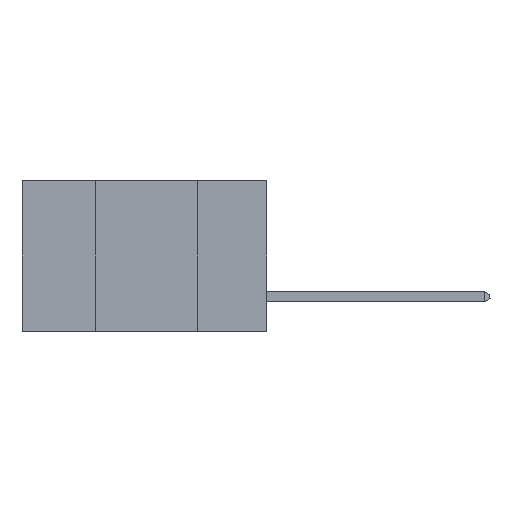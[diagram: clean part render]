
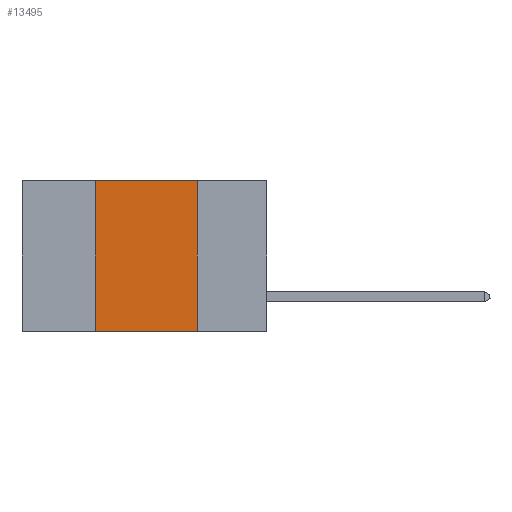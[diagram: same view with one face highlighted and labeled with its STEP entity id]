
A CAD part, left-side view. The second image highlights one B-rep face of the part: STEP entity #13495.
In plain terms, the highlighted planar face has unit normal (-1, 0, 0).
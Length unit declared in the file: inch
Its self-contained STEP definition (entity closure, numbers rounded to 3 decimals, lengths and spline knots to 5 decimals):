
#2422 = LINE ( 'NONE', #14646, #25471 ) ;
#2868 = CARTESIAN_POINT ( 'NONE',  ( 0., 0.42, 0. ) ) ;
#5227 = DIRECTION ( 'NONE',  ( 0., 0., -1. ) ) ;
#6954 = ORIENTED_EDGE ( 'NONE', *, *, #23895, .F. ) ;
#7802 = VERTEX_POINT ( 'NONE', #35195 ) ;
#7934 = EDGE_CURVE ( 'NONE', #14962, #7802, #11717, .T. ) ;
#8700 = DIRECTION ( 'NONE',  ( 0., 0., -1. ) ) ;
#10096 = CARTESIAN_POINT ( 'NONE',  ( 0., 0.42, -0.37 ) ) ;
#11717 = LINE ( 'NONE', #23945, #12528 ) ;
#12528 = VECTOR ( 'NONE', #8700, 39.37008 ) ;
#13495 = ADVANCED_FACE ( 'NONE', ( #26671 ), #35683, .F. ) ;
#14646 = CARTESIAN_POINT ( 'NONE',  ( 0., 0.6, 0. ) ) ;
#14962 = VERTEX_POINT ( 'NONE', #21845 ) ;
#15975 = LINE ( 'NONE', #31417, #37456 ) ;
#17868 = CARTESIAN_POINT ( 'NONE',  ( 0., 0.42, 0. ) ) ;
#18781 = DIRECTION ( 'NONE',  ( 0., -1., 0. ) ) ;
#21075 = DIRECTION ( 'NONE',  ( 0., 0., 1. ) ) ;
#21845 = CARTESIAN_POINT ( 'NONE',  ( 0., 0.17, 0. ) ) ;
#22708 = EDGE_CURVE ( 'NONE', #36100, #7802, #15975, .T. ) ;
#23895 = EDGE_CURVE ( 'NONE', #38594, #14962, #2422, .T. ) ;
#23945 = CARTESIAN_POINT ( 'NONE',  ( 0., 0.17, 0. ) ) ;
#24073 = LINE ( 'NONE', #17868, #25766 ) ;
#25471 = VECTOR ( 'NONE', #26886, 39.37008 ) ;
#25766 = VECTOR ( 'NONE', #21075, 39.37008 ) ;
#26671 = FACE_OUTER_BOUND ( 'NONE', #33852, .T. ) ;
#26886 = DIRECTION ( 'NONE',  ( 0., -1., 0. ) ) ;
#26967 = ORIENTED_EDGE ( 'NONE', *, *, #7934, .F. ) ;
#29677 = CARTESIAN_POINT ( 'NONE',  ( 0., 0.6, 0. ) ) ;
#30968 = ORIENTED_EDGE ( 'NONE', *, *, #22708, .T. ) ;
#31417 = CARTESIAN_POINT ( 'NONE',  ( 0., 0.6, -0.37 ) ) ;
#33852 = EDGE_LOOP ( 'NONE', ( #26967, #6954, #39595, #30968 ) ) ;
#35195 = CARTESIAN_POINT ( 'NONE',  ( 0., 0.17, -0.37 ) ) ;
#35683 = PLANE ( 'NONE',  #39600 ) ;
#35886 = DIRECTION ( 'NONE',  ( 1., 0., 0. ) ) ;
#36100 = VERTEX_POINT ( 'NONE', #10096 ) ;
#37456 = VECTOR ( 'NONE', #18781, 39.37008 ) ;
#38594 = VERTEX_POINT ( 'NONE', #2868 ) ;
#38949 = EDGE_CURVE ( 'NONE', #36100, #38594, #24073, .T. ) ;
#39595 = ORIENTED_EDGE ( 'NONE', *, *, #38949, .F. ) ;
#39600 = AXIS2_PLACEMENT_3D ( 'NONE', #29677, #35886, #5227 ) ;
